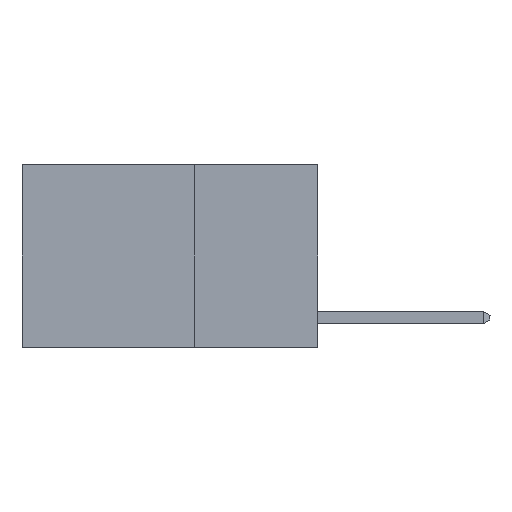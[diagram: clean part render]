
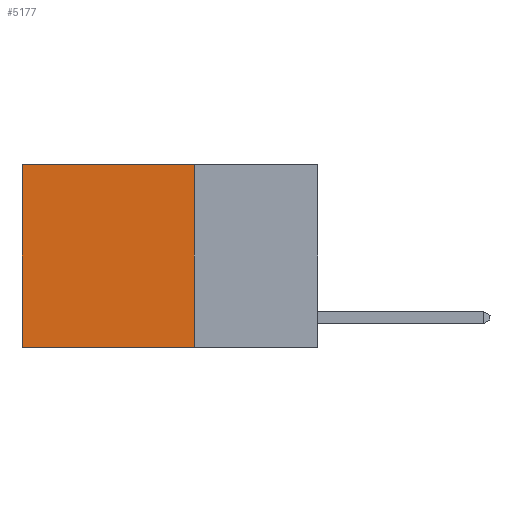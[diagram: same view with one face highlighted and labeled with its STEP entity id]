
A CAD part, left-side view. The second image highlights one B-rep face of the part: STEP entity #5177.
In plain terms, the highlighted planar face has unit normal (-1, 0, 0).
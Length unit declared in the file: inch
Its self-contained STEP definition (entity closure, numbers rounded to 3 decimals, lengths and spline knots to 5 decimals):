
#131 = EDGE_CURVE ( 'NONE', #1165, #13386, #2667, .T. ) ;
#1165 = VERTEX_POINT ( 'NONE', #5831 ) ;
#1296 = EDGE_CURVE ( 'NONE', #12301, #13386, #11399, .T. ) ;
#1438 = AXIS2_PLACEMENT_3D ( 'NONE', #2019, #4525, #4590 ) ;
#1862 = LINE ( 'NONE', #8086, #7356 ) ;
#2019 = CARTESIAN_POINT ( 'NONE',  ( 0.2625, 0.25, 0. ) ) ;
#2285 = ORIENTED_EDGE ( 'NONE', *, *, #13067, .T. ) ;
#2498 = DIRECTION ( 'NONE',  ( 0., 0., -1. ) ) ;
#2546 = CARTESIAN_POINT ( 'NONE',  ( 0.2625, 0.6, -0.37 ) ) ;
#2667 = LINE ( 'NONE', #9892, #5165 ) ;
#3252 = VERTEX_POINT ( 'NONE', #8193 ) ;
#3993 = VECTOR ( 'NONE', #7325, 39.37008 ) ;
#4525 = DIRECTION ( 'NONE',  ( 1., 0., 0. ) ) ;
#4590 = DIRECTION ( 'NONE',  ( 0., 0., -1. ) ) ;
#4682 = PLANE ( 'NONE',  #1438 ) ;
#5165 = VECTOR ( 'NONE', #2498, 39.37008 ) ;
#5177 = ADVANCED_FACE ( 'NONE', ( #11208 ), #4682, .F. ) ;
#5624 = VECTOR ( 'NONE', #12918, 39.37008 ) ;
#5831 = CARTESIAN_POINT ( 'NONE',  ( 0.2625, 0.6, 0. ) ) ;
#6255 = ORIENTED_EDGE ( 'NONE', *, *, #131, .T. ) ;
#7209 = ORIENTED_EDGE ( 'NONE', *, *, #1296, .F. ) ;
#7325 = DIRECTION ( 'NONE',  ( 0., 0., -1. ) ) ;
#7356 = VECTOR ( 'NONE', #10166, 39.37008 ) ;
#8086 = CARTESIAN_POINT ( 'NONE',  ( 0.2625, 0.25, 0. ) ) ;
#8193 = CARTESIAN_POINT ( 'NONE',  ( 0.2625, 0.25, 0. ) ) ;
#9615 = EDGE_CURVE ( 'NONE', #3252, #12301, #9867, .T. ) ;
#9867 = LINE ( 'NONE', #13310, #3993 ) ;
#9892 = CARTESIAN_POINT ( 'NONE',  ( 0.2625, 0.6, 0. ) ) ;
#10166 = DIRECTION ( 'NONE',  ( 0., 1., 0. ) ) ;
#11208 = FACE_OUTER_BOUND ( 'NONE', #12387, .T. ) ;
#11245 = ORIENTED_EDGE ( 'NONE', *, *, #9615, .F. ) ;
#11399 = LINE ( 'NONE', #12963, #5624 ) ;
#12301 = VERTEX_POINT ( 'NONE', #12847 ) ;
#12387 = EDGE_LOOP ( 'NONE', ( #6255, #7209, #11245, #2285 ) ) ;
#12847 = CARTESIAN_POINT ( 'NONE',  ( 0.2625, 0.25, -0.37 ) ) ;
#12918 = DIRECTION ( 'NONE',  ( 0., 1., 0. ) ) ;
#12963 = CARTESIAN_POINT ( 'NONE',  ( 0.2625, 0.25, -0.37 ) ) ;
#13067 = EDGE_CURVE ( 'NONE', #3252, #1165, #1862, .T. ) ;
#13310 = CARTESIAN_POINT ( 'NONE',  ( 0.2625, 0.25, 0. ) ) ;
#13386 = VERTEX_POINT ( 'NONE', #2546 ) ;
